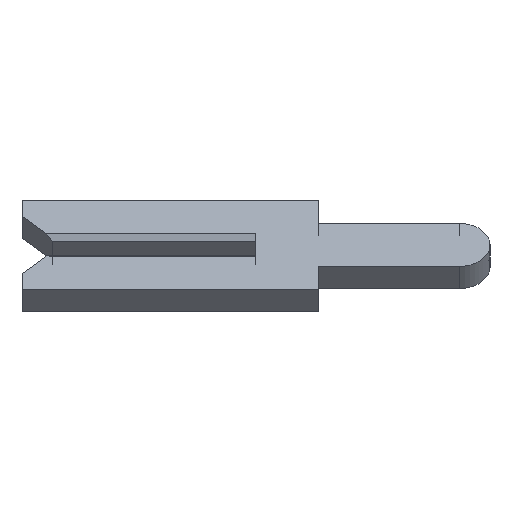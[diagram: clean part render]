
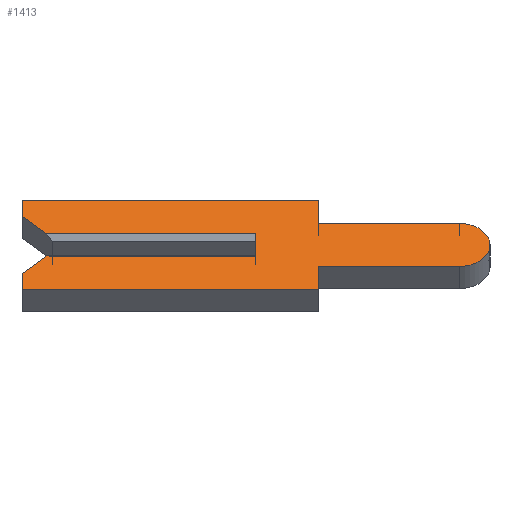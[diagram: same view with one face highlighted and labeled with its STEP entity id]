
A CAD part, left-side view. The second image highlights one B-rep face of the part: STEP entity #1413.
In plain terms, the highlighted face is planar.
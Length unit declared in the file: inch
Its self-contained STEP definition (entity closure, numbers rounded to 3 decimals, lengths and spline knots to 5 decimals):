
#10 = ORIENTED_EDGE ( 'NONE', *, *, #923, .F. ) ;
#12 = LINE ( 'NONE', #143, #1296 ) ;
#97 = EDGE_CURVE ( 'NONE', #1818, #1133, #133, .T. ) ;
#104 = CARTESIAN_POINT ( 'NONE',  ( -0.01, -0.04, 0.04 ) ) ;
#106 = VECTOR ( 'NONE', #1739, 39.37008 ) ;
#133 = LINE ( 'NONE', #104, #1369 ) ;
#143 = CARTESIAN_POINT ( 'NONE',  ( -0.01, 0., 0.0065 ) ) ;
#150 = DIRECTION ( 'NONE',  ( 0., -1., 0. ) ) ;
#173 = CARTESIAN_POINT ( 'NONE',  ( -0.01, 0.134, 0.01 ) ) ;
#179 = EDGE_CURVE ( 'NONE', #1281, #500, #712, .T. ) ;
#195 = CARTESIAN_POINT ( 'NONE',  ( -0.01, 0., 0.01 ) ) ;
#202 = AXIS2_PLACEMENT_3D ( 'NONE', #1237, #1569, #1057 ) ;
#252 = ORIENTED_EDGE ( 'NONE', *, *, #1808, .F. ) ;
#257 = EDGE_CURVE ( 'NONE', #1790, #1281, #867, .T. ) ;
#276 = CARTESIAN_POINT ( 'NONE',  ( -0.01, 0.134, -0.01 ) ) ;
#282 = CARTESIAN_POINT ( 'NONE',  ( -0.01, -0.1305, -0.0195 ) ) ;
#288 = VECTOR ( 'NONE', #1803, 39.37008 ) ;
#290 = CARTESIAN_POINT ( 'NONE',  ( -0.01, 0.15, -0.04 ) ) ;
#342 = VECTOR ( 'NONE', #1854, 39.37008 ) ;
#349 = FACE_OUTER_BOUND ( 'NONE', #1875, .T. ) ;
#353 = CARTESIAN_POINT ( 'NONE',  ( -0.01, 0.15, -0.026 ) ) ;
#380 = DIRECTION ( 'NONE',  ( 0., 0.707, 0.707 ) ) ;
#393 = VECTOR ( 'NONE', #826, 39.37008 ) ;
#419 = EDGE_CURVE ( 'NONE', #767, #967, #1964, .T. ) ;
#427 = LINE ( 'NONE', #1882, #1002 ) ;
#430 = VERTEX_POINT ( 'NONE', #1994 ) ;
#454 = ORIENTED_EDGE ( 'NONE', *, *, #179, .F. ) ;
#459 = LINE ( 'NONE', #2118, #1879 ) ;
#463 = CARTESIAN_POINT ( 'NONE',  ( -0.01, -0.04, 0.04 ) ) ;
#470 = DIRECTION ( 'NONE',  ( 0., -1., 0. ) ) ;
#479 = CARTESIAN_POINT ( 'NONE',  ( -0.01, -0.04, -0.04 ) ) ;
#500 = VERTEX_POINT ( 'NONE', #479 ) ;
#569 = CARTESIAN_POINT ( 'NONE',  ( -0.01, 0.15, 0.026 ) ) ;
#591 = ORIENTED_EDGE ( 'NONE', *, *, #1487, .F. ) ;
#612 = ORIENTED_EDGE ( 'NONE', *, *, #257, .F. ) ;
#616 = EDGE_CURVE ( 'NONE', #1133, #1211, #1096, .T. ) ;
#628 = EDGE_CURVE ( 'NONE', #1211, #1790, #762, .T. ) ;
#637 = CARTESIAN_POINT ( 'NONE',  ( -0.01, 0.15, 0.01 ) ) ;
#662 = DIRECTION ( 'NONE',  ( 0., 0., -1. ) ) ;
#704 = CARTESIAN_POINT ( 'NONE',  ( -0.01, -0.04, 0.0195 ) ) ;
#712 = LINE ( 'NONE', #953, #1498 ) ;
#718 = ORIENTED_EDGE ( 'NONE', *, *, #97, .F. ) ;
#725 = VECTOR ( 'NONE', #1449, 39.37008 ) ;
#743 = CARTESIAN_POINT ( 'NONE',  ( -0.01, 0.1305, -0.0065 ) ) ;
#762 = CIRCLE ( 'NONE', #2123, 0.0195 ) ;
#767 = VERTEX_POINT ( 'NONE', #173 ) ;
#826 = DIRECTION ( 'NONE',  ( 0., 0., 1. ) ) ;
#867 = LINE ( 'NONE', #1637, #288 ) ;
#869 = ORIENTED_EDGE ( 'NONE', *, *, #2098, .F. ) ;
#882 = EDGE_CURVE ( 'NONE', #1765, #1894, #1231, .T. ) ;
#894 = PLANE ( 'NONE',  #202 ) ;
#923 = EDGE_CURVE ( 'NONE', #430, #1708, #1960, .T. ) ;
#926 = VERTEX_POINT ( 'NONE', #1008 ) ;
#953 = CARTESIAN_POINT ( 'NONE',  ( -0.01, -0.04, -0.04 ) ) ;
#967 = VERTEX_POINT ( 'NONE', #195 ) ;
#992 = VECTOR ( 'NONE', #470, 39.37008 ) ;
#1002 = VECTOR ( 'NONE', #380, 39.37008 ) ;
#1008 = CARTESIAN_POINT ( 'NONE',  ( -0.01, 0.15, 0.026 ) ) ;
#1056 = LINE ( 'NONE', #290, #725 ) ;
#1057 = DIRECTION ( 'NONE',  ( 0., 0., -1. ) ) ;
#1096 = LINE ( 'NONE', #704, #992 ) ;
#1103 = DIRECTION ( 'NONE',  ( 0., 0., -1. ) ) ;
#1105 = ORIENTED_EDGE ( 'NONE', *, *, #419, .T. ) ;
#1133 = VERTEX_POINT ( 'NONE', #1562 ) ;
#1142 = EDGE_CURVE ( 'NONE', #767, #926, #427, .T. ) ;
#1156 = ORIENTED_EDGE ( 'NONE', *, *, #1142, .F. ) ;
#1193 = CARTESIAN_POINT ( 'NONE',  ( -0.01, -0.1305, -0.01 ) ) ;
#1209 = VERTEX_POINT ( 'NONE', #2066 ) ;
#1211 = VERTEX_POINT ( 'NONE', #1401 ) ;
#1231 = LINE ( 'NONE', #1193, #342 ) ;
#1237 = CARTESIAN_POINT ( 'NONE',  ( -0.01, -0.1305, 0. ) ) ;
#1281 = VERTEX_POINT ( 'NONE', #1715 ) ;
#1296 = VECTOR ( 'NONE', #1470, 39.37008 ) ;
#1369 = VECTOR ( 'NONE', #1788, 39.37008 ) ;
#1374 = ORIENTED_EDGE ( 'NONE', *, *, #1777, .F. ) ;
#1379 = VECTOR ( 'NONE', #1916, 39.37008 ) ;
#1396 = ORIENTED_EDGE ( 'NONE', *, *, #1680, .F. ) ;
#1401 = CARTESIAN_POINT ( 'NONE',  ( -0.01, -0.1305, 0.0195 ) ) ;
#1413 = ADVANCED_FACE ( 'NONE', ( #349 ), #894, .F. ) ;
#1430 = ORIENTED_EDGE ( 'NONE', *, *, #628, .F. ) ;
#1449 = DIRECTION ( 'NONE',  ( 0., 1., 0. ) ) ;
#1462 = CARTESIAN_POINT ( 'NONE',  ( -0.01, 0.15, -0.026 ) ) ;
#1470 = DIRECTION ( 'NONE',  ( 0., 0., 1. ) ) ;
#1487 = EDGE_CURVE ( 'NONE', #926, #1209, #1527, .T. ) ;
#1497 = CARTESIAN_POINT ( 'NONE',  ( -0.01, -0.1305, 0. ) ) ;
#1498 = VECTOR ( 'NONE', #1103, 39.37008 ) ;
#1506 = ORIENTED_EDGE ( 'NONE', *, *, #616, .F. ) ;
#1527 = LINE ( 'NONE', #569, #106 ) ;
#1549 = VECTOR ( 'NONE', #150, 39.37008 ) ;
#1562 = CARTESIAN_POINT ( 'NONE',  ( -0.01, -0.04, 0.0195 ) ) ;
#1569 = DIRECTION ( 'NONE',  ( 1., 0., 0. ) ) ;
#1637 = CARTESIAN_POINT ( 'NONE',  ( -0.01, -0.04, -0.0195 ) ) ;
#1664 = DIRECTION ( 'NONE',  ( 1., 0., 0. ) ) ;
#1680 = EDGE_CURVE ( 'NONE', #1708, #1765, #1691, .T. ) ;
#1691 = LINE ( 'NONE', #743, #1379 ) ;
#1708 = VERTEX_POINT ( 'NONE', #1462 ) ;
#1715 = CARTESIAN_POINT ( 'NONE',  ( -0.01, -0.04, -0.0195 ) ) ;
#1739 = DIRECTION ( 'NONE',  ( 0., 0., 1. ) ) ;
#1765 = VERTEX_POINT ( 'NONE', #276 ) ;
#1777 = EDGE_CURVE ( 'NONE', #500, #430, #1056, .T. ) ;
#1785 = DIRECTION ( 'NONE',  ( 0., -1., 0. ) ) ;
#1788 = DIRECTION ( 'NONE',  ( 0., 0., -1. ) ) ;
#1790 = VERTEX_POINT ( 'NONE', #282 ) ;
#1803 = DIRECTION ( 'NONE',  ( 0., 1., 0. ) ) ;
#1808 = EDGE_CURVE ( 'NONE', #1209, #1818, #459, .T. ) ;
#1818 = VERTEX_POINT ( 'NONE', #463 ) ;
#1854 = DIRECTION ( 'NONE',  ( 0., -1., 0. ) ) ;
#1875 = EDGE_LOOP ( 'NONE', ( #1105, #869, #1947, #1396, #10, #1374, #454, #612, #1430, #1506, #718, #252, #591, #1156 ) ) ;
#1879 = VECTOR ( 'NONE', #1785, 39.37008 ) ;
#1882 = CARTESIAN_POINT ( 'NONE',  ( -0.01, 0.1305, 0.0065 ) ) ;
#1894 = VERTEX_POINT ( 'NONE', #1965 ) ;
#1916 = DIRECTION ( 'NONE',  ( 0., -0.707, 0.707 ) ) ;
#1947 = ORIENTED_EDGE ( 'NONE', *, *, #882, .F. ) ;
#1960 = LINE ( 'NONE', #353, #393 ) ;
#1964 = LINE ( 'NONE', #637, #1549 ) ;
#1965 = CARTESIAN_POINT ( 'NONE',  ( -0.01, 0., -0.01 ) ) ;
#1994 = CARTESIAN_POINT ( 'NONE',  ( -0.01, 0.15, -0.04 ) ) ;
#2066 = CARTESIAN_POINT ( 'NONE',  ( -0.01, 0.15, 0.04 ) ) ;
#2098 = EDGE_CURVE ( 'NONE', #1894, #967, #12, .T. ) ;
#2118 = CARTESIAN_POINT ( 'NONE',  ( -0.01, 0.15, 0.04 ) ) ;
#2123 = AXIS2_PLACEMENT_3D ( 'NONE', #1497, #1664, #662 ) ;
